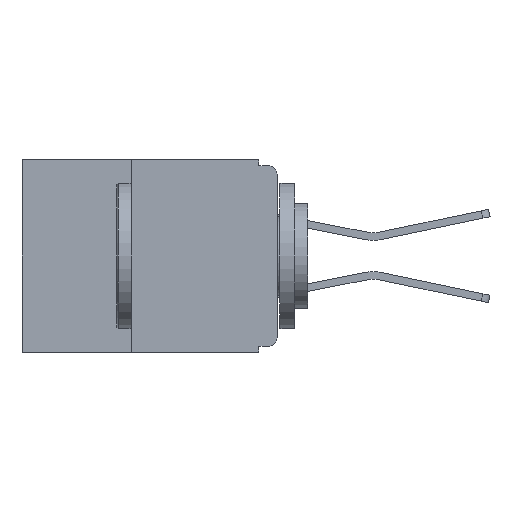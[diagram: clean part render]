
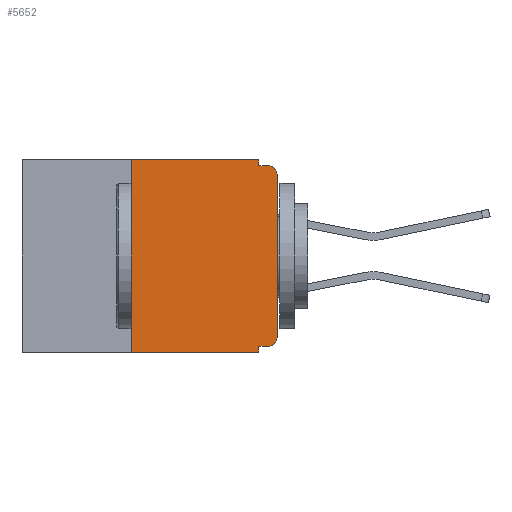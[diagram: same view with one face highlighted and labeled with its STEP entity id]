
A CAD part, left-side view. The second image highlights one B-rep face of the part: STEP entity #5652.
In plain terms, the highlighted planar face has unit normal (-1, 0, 0).
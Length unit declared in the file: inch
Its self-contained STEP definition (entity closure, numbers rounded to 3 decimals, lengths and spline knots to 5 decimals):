
#377 = CARTESIAN_POINT ( 'NONE',  ( 0., 0.437, 0. ) ) ;
#397 = ORIENTED_EDGE ( 'NONE', *, *, #4780, .T. ) ;
#711 = ORIENTED_EDGE ( 'NONE', *, *, #19910, .F. ) ;
#1170 = VECTOR ( 'NONE', #1606, 39.37008 ) ;
#1606 = DIRECTION ( 'NONE',  ( 0., 0., 1. ) ) ;
#1750 = CARTESIAN_POINT ( 'NONE',  ( 0., 0., 0. ) ) ;
#1757 = EDGE_CURVE ( 'NONE', #17253, #2712, #5317, .T. ) ;
#1913 = VERTEX_POINT ( 'NONE', #24222 ) ;
#1923 = ORIENTED_EDGE ( 'NONE', *, *, #4401, .F. ) ;
#2191 = CARTESIAN_POINT ( 'NONE',  ( 0., 0.031, 0. ) ) ;
#2712 = VERTEX_POINT ( 'NONE', #19445 ) ;
#2860 = VERTEX_POINT ( 'NONE', #25518 ) ;
#2898 = VECTOR ( 'NONE', #24206, 39.37008 ) ;
#3129 = VECTOR ( 'NONE', #16243, 39.37008 ) ;
#3276 = VECTOR ( 'NONE', #4262, 39.37008 ) ;
#3398 = ORIENTED_EDGE ( 'NONE', *, *, #14402, .T. ) ;
#3696 = ORIENTED_EDGE ( 'NONE', *, *, #4770, .F. ) ;
#3777 = EDGE_CURVE ( 'NONE', #21187, #3828, #7471, .T. ) ;
#3791 = LINE ( 'NONE', #22213, #3129 ) ;
#3828 = VERTEX_POINT ( 'NONE', #12132 ) ;
#4262 = DIRECTION ( 'NONE',  ( 0., 0., -1. ) ) ;
#4401 = EDGE_CURVE ( 'NONE', #21187, #17253, #13779, .T. ) ;
#4770 = EDGE_CURVE ( 'NONE', #6797, #1913, #20396, .T. ) ;
#4780 = EDGE_CURVE ( 'NONE', #14261, #1913, #9680, .T. ) ;
#4830 = ORIENTED_EDGE ( 'NONE', *, *, #1757, .F. ) ;
#5317 = LINE ( 'NONE', #25684, #15475 ) ;
#5468 = ORIENTED_EDGE ( 'NONE', *, *, #3777, .T. ) ;
#5652 = ADVANCED_FACE ( 'NONE', ( #20961 ), #20101, .F. ) ;
#5741 = DIRECTION ( 'NONE',  ( 0., 0., -1. ) ) ;
#5977 = CARTESIAN_POINT ( 'NONE',  ( 0., 0.031, -0.01 ) ) ;
#6031 = LINE ( 'NONE', #1750, #1170 ) ;
#6797 = VERTEX_POINT ( 'NONE', #5977 ) ;
#7471 = CIRCLE ( 'NONE', #17216, 0.015 ) ;
#7788 = EDGE_CURVE ( 'NONE', #3828, #14261, #6031, .T. ) ;
#9374 = DIRECTION ( 'NONE',  ( 0., 0., -1. ) ) ;
#9661 = DIRECTION ( 'NONE',  ( -1., 0., 0. ) ) ;
#9680 = CIRCLE ( 'NONE', #17057, 0.015 ) ;
#9749 = LINE ( 'NONE', #17020, #19850 ) ;
#9911 = CARTESIAN_POINT ( 'NONE',  ( 0., 0.015, -0.025 ) ) ;
#10320 = DIRECTION ( 'NONE',  ( 0., -1., 0. ) ) ;
#10379 = CARTESIAN_POINT ( 'NONE',  ( 0., 0., -0.01 ) ) ;
#10735 = ORIENTED_EDGE ( 'NONE', *, *, #12861, .F. ) ;
#10883 = CARTESIAN_POINT ( 'NONE',  ( 0., 0.25, -0.33 ) ) ;
#12132 = CARTESIAN_POINT ( 'NONE',  ( 0., 0., -0.305 ) ) ;
#12634 = CARTESIAN_POINT ( 'NONE',  ( 0., 0., -0.025 ) ) ;
#12861 = EDGE_CURVE ( 'NONE', #25153, #17719, #3791, .T. ) ;
#13196 = LINE ( 'NONE', #377, #24479 ) ;
#13391 = DIRECTION ( 'NONE',  ( 0., 0., -1. ) ) ;
#13397 = DIRECTION ( 'NONE',  ( -1., 0., 0. ) ) ;
#13450 = CARTESIAN_POINT ( 'NONE',  ( 0., 0.015, -0.305 ) ) ;
#13779 = LINE ( 'NONE', #23403, #2898 ) ;
#14137 = LINE ( 'NONE', #2191, #3276 ) ;
#14261 = VERTEX_POINT ( 'NONE', #12634 ) ;
#14402 = EDGE_CURVE ( 'NONE', #25153, #2712, #9749, .T. ) ;
#15077 = DIRECTION ( 'NONE',  ( 0., -1., 0. ) ) ;
#15133 = ORIENTED_EDGE ( 'NONE', *, *, #7788, .T. ) ;
#15349 = EDGE_CURVE ( 'NONE', #2860, #6797, #14137, .T. ) ;
#15475 = VECTOR ( 'NONE', #5741, 39.37008 ) ;
#16243 = DIRECTION ( 'NONE',  ( 0., 0., 1. ) ) ;
#16642 = CARTESIAN_POINT ( 'NONE',  ( 0., 0.015, -0.32 ) ) ;
#17020 = CARTESIAN_POINT ( 'NONE',  ( 0., 0.437, -0.33 ) ) ;
#17057 = AXIS2_PLACEMENT_3D ( 'NONE', #9911, #9661, #9374 ) ;
#17216 = AXIS2_PLACEMENT_3D ( 'NONE', #13450, #13397, #13391 ) ;
#17253 = VERTEX_POINT ( 'NONE', #24377 ) ;
#17719 = VERTEX_POINT ( 'NONE', #25885 ) ;
#19445 = CARTESIAN_POINT ( 'NONE',  ( 0., 0.031, -0.33 ) ) ;
#19776 = VECTOR ( 'NONE', #10320, 39.37008 ) ;
#19850 = VECTOR ( 'NONE', #15077, 39.37008 ) ;
#19910 = EDGE_CURVE ( 'NONE', #17719, #2860, #13196, .T. ) ;
#19955 = DIRECTION ( 'NONE',  ( 0., 0., -1. ) ) ;
#19979 = DIRECTION ( 'NONE',  ( 1., 0., 0. ) ) ;
#20046 = CARTESIAN_POINT ( 'NONE',  ( 0., 0.437, 0. ) ) ;
#20101 = PLANE ( 'NONE',  #20962 ) ;
#20396 = LINE ( 'NONE', #10379, #19776 ) ;
#20787 = DIRECTION ( 'NONE',  ( 0., -1., 0. ) ) ;
#20961 = FACE_OUTER_BOUND ( 'NONE', #21902, .T. ) ;
#20962 = AXIS2_PLACEMENT_3D ( 'NONE', #20046, #19979, #19955 ) ;
#21187 = VERTEX_POINT ( 'NONE', #16642 ) ;
#21902 = EDGE_LOOP ( 'NONE', ( #15133, #397, #3696, #26177, #711, #10735, #3398, #4830, #1923, #5468 ) ) ;
#22213 = CARTESIAN_POINT ( 'NONE',  ( 0., 0.25, -0.33 ) ) ;
#23403 = CARTESIAN_POINT ( 'NONE',  ( 0., 0., -0.32 ) ) ;
#24206 = DIRECTION ( 'NONE',  ( 0., 1., 0. ) ) ;
#24222 = CARTESIAN_POINT ( 'NONE',  ( 0., 0.015, -0.01 ) ) ;
#24377 = CARTESIAN_POINT ( 'NONE',  ( 0., 0.031, -0.32 ) ) ;
#24479 = VECTOR ( 'NONE', #20787, 39.37008 ) ;
#25153 = VERTEX_POINT ( 'NONE', #10883 ) ;
#25518 = CARTESIAN_POINT ( 'NONE',  ( 0., 0.031, 0. ) ) ;
#25684 = CARTESIAN_POINT ( 'NONE',  ( 0., 0.031, -0.33 ) ) ;
#25885 = CARTESIAN_POINT ( 'NONE',  ( 0., 0.25, 0. ) ) ;
#26177 = ORIENTED_EDGE ( 'NONE', *, *, #15349, .F. ) ;
